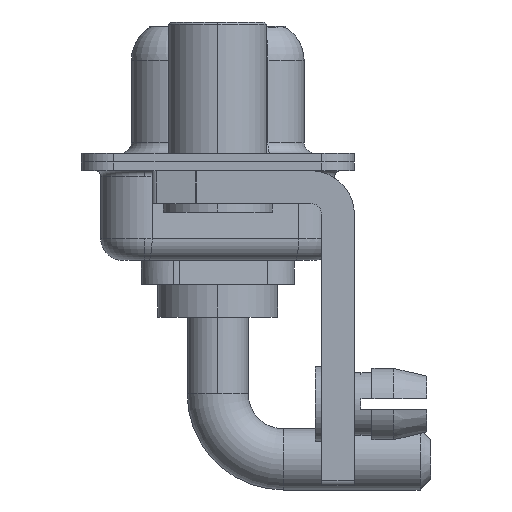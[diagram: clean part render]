
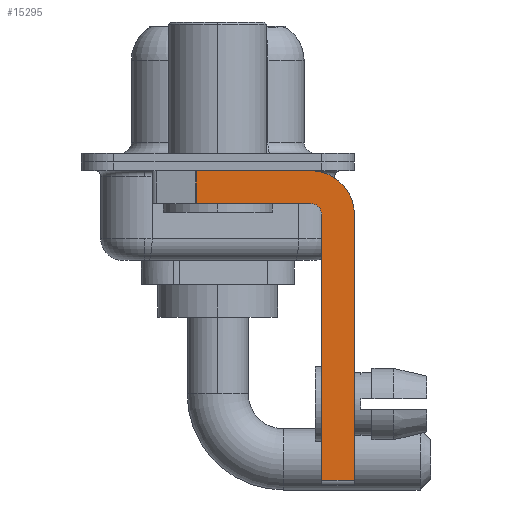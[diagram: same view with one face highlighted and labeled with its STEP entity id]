
A CAD part, left-side view. The second image highlights one B-rep face of the part: STEP entity #15295.
In plain terms, the highlighted planar face has unit normal (-1, 0, 0).
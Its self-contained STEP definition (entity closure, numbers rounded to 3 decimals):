
#123 = ORIENTED_EDGE ( 'NONE', *, *, #4072, .F. ) ;
#260 = CARTESIAN_POINT ( 'NONE',  ( -2.9, -4.75, -14.8 ) ) ;
#335 = CARTESIAN_POINT ( 'NONE',  ( -2.9, -4.25, -1.9 ) ) ;
#838 = DIRECTION ( 'NONE',  ( 0., 0., -1. ) ) ;
#1735 = DIRECTION ( 'NONE',  ( 0., 1., 0. ) ) ;
#2059 = ORIENTED_EDGE ( 'NONE', *, *, #16193, .F. ) ;
#2238 = CARTESIAN_POINT ( 'NONE',  ( -2.9, 0.978, -1.9 ) ) ;
#2450 = DIRECTION ( 'NONE',  ( 0., -1., 0. ) ) ;
#2843 = CARTESIAN_POINT ( 'NONE',  ( -2.9, -6.25, -2.4 ) ) ;
#3131 = DIRECTION ( 'NONE',  ( 0., -1., 0. ) ) ;
#3331 = VECTOR ( 'NONE', #5638, 1000. ) ;
#3344 = ORIENTED_EDGE ( 'NONE', *, *, #12958, .F. ) ;
#3497 = LINE ( 'NONE', #10301, #4958 ) ;
#3616 = VERTEX_POINT ( 'NONE', #14939 ) ;
#3735 = VECTOR ( 'NONE', #2450, 1000. ) ;
#4072 = EDGE_CURVE ( 'NONE', #7972, #8576, #10212, .T. ) ;
#4197 = VECTOR ( 'NONE', #8513, 1000. ) ;
#4384 = VERTEX_POINT ( 'NONE', #17107 ) ;
#4958 = VECTOR ( 'NONE', #8897, 1000. ) ;
#4961 = VERTEX_POINT ( 'NONE', #6417 ) ;
#4962 = EDGE_CURVE ( 'NONE', #4384, #7972, #11780, .T. ) ;
#5638 = DIRECTION ( 'NONE',  ( 0., 0., 1. ) ) ;
#5700 = CIRCLE ( 'NONE', #15286, 0.5 ) ;
#5719 = EDGE_LOOP ( 'NONE', ( #17127, #13753, #2059, #8638, #11628, #9675, #3344, #123 ) ) ;
#5725 = LINE ( 'NONE', #260, #3331 ) ;
#5771 = LINE ( 'NONE', #13882, #9714 ) ;
#6130 = FACE_OUTER_BOUND ( 'NONE', #5719, .T. ) ;
#6417 = CARTESIAN_POINT ( 'NONE',  ( -2.9, -4.75, -2.4 ) ) ;
#7097 = LINE ( 'NONE', #13697, #4197 ) ;
#7972 = VERTEX_POINT ( 'NONE', #9636 ) ;
#8129 = CARTESIAN_POINT ( 'NONE',  ( -2.9, -4.25, -2.4 ) ) ;
#8395 = DIRECTION ( 'NONE',  ( 0., 0., -1. ) ) ;
#8513 = DIRECTION ( 'NONE',  ( 0., 0., -1. ) ) ;
#8576 = VERTEX_POINT ( 'NONE', #2843 ) ;
#8638 = ORIENTED_EDGE ( 'NONE', *, *, #8949, .F. ) ;
#8897 = DIRECTION ( 'NONE',  ( 0., 0., -1. ) ) ;
#8949 = EDGE_CURVE ( 'NONE', #4961, #3616, #5700, .T. ) ;
#9574 = CARTESIAN_POINT ( 'NONE',  ( -2.9, -6.25, -14.55 ) ) ;
#9636 = CARTESIAN_POINT ( 'NONE',  ( -2.9, -4.25, -0.4 ) ) ;
#9675 = ORIENTED_EDGE ( 'NONE', *, *, #11082, .T. ) ;
#9714 = VECTOR ( 'NONE', #3131, 1000. ) ;
#9858 = LINE ( 'NONE', #335, #14536 ) ;
#10212 = CIRCLE ( 'NONE', #14431, 2. ) ;
#10301 = CARTESIAN_POINT ( 'NONE',  ( -2.9, 0.978, -1.9 ) ) ;
#10507 = DIRECTION ( 'NONE',  ( 0., 0., 1. ) ) ;
#10835 = AXIS2_PLACEMENT_3D ( 'NONE', #13982, #12904, #838 ) ;
#11082 = EDGE_CURVE ( 'NONE', #14316, #12424, #5771, .T. ) ;
#11216 = VERTEX_POINT ( 'NONE', #2238 ) ;
#11398 = EDGE_CURVE ( 'NONE', #14316, #4961, #5725, .T. ) ;
#11498 = PLANE ( 'NONE',  #10835 ) ;
#11628 = ORIENTED_EDGE ( 'NONE', *, *, #11398, .F. ) ;
#11780 = LINE ( 'NONE', #14540, #3735 ) ;
#12424 = VERTEX_POINT ( 'NONE', #9574 ) ;
#12904 = DIRECTION ( 'NONE',  ( 1., 0., 0. ) ) ;
#12958 = EDGE_CURVE ( 'NONE', #8576, #12424, #7097, .T. ) ;
#13697 = CARTESIAN_POINT ( 'NONE',  ( -2.9, -6.25, -2.4 ) ) ;
#13753 = ORIENTED_EDGE ( 'NONE', *, *, #16355, .T. ) ;
#13882 = CARTESIAN_POINT ( 'NONE',  ( -2.9, -4.25, -14.55 ) ) ;
#13982 = CARTESIAN_POINT ( 'NONE',  ( -2.9, -4.25, -2.4 ) ) ;
#14219 = DIRECTION ( 'NONE',  ( -1., 0., 0. ) ) ;
#14316 = VERTEX_POINT ( 'NONE', #16415 ) ;
#14431 = AXIS2_PLACEMENT_3D ( 'NONE', #8129, #14912, #8395 ) ;
#14536 = VECTOR ( 'NONE', #1735, 1000. ) ;
#14540 = CARTESIAN_POINT ( 'NONE',  ( -2.9, 3., -0.4 ) ) ;
#14912 = DIRECTION ( 'NONE',  ( 1., 0., 0. ) ) ;
#14939 = CARTESIAN_POINT ( 'NONE',  ( -2.9, -4.25, -1.9 ) ) ;
#15286 = AXIS2_PLACEMENT_3D ( 'NONE', #16853, #14219, #10507 ) ;
#15295 = ADVANCED_FACE ( 'NONE', ( #6130 ), #11498, .F. ) ;
#16193 = EDGE_CURVE ( 'NONE', #3616, #11216, #9858, .T. ) ;
#16355 = EDGE_CURVE ( 'NONE', #4384, #11216, #3497, .T. ) ;
#16415 = CARTESIAN_POINT ( 'NONE',  ( -2.9, -4.75, -14.55 ) ) ;
#16853 = CARTESIAN_POINT ( 'NONE',  ( -2.9, -4.25, -2.4 ) ) ;
#17107 = CARTESIAN_POINT ( 'NONE',  ( -2.9, 0.978, -0.4 ) ) ;
#17127 = ORIENTED_EDGE ( 'NONE', *, *, #4962, .F. ) ;
